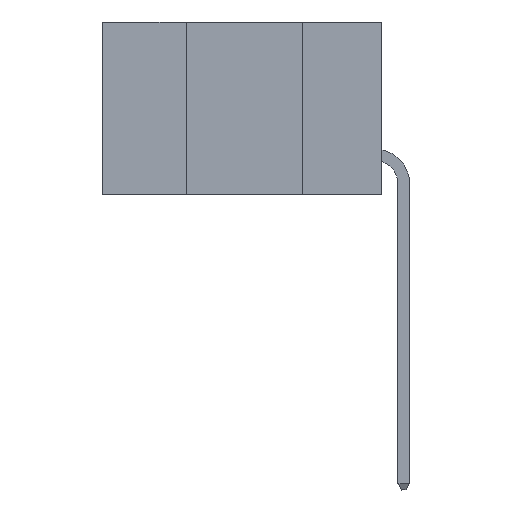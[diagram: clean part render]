
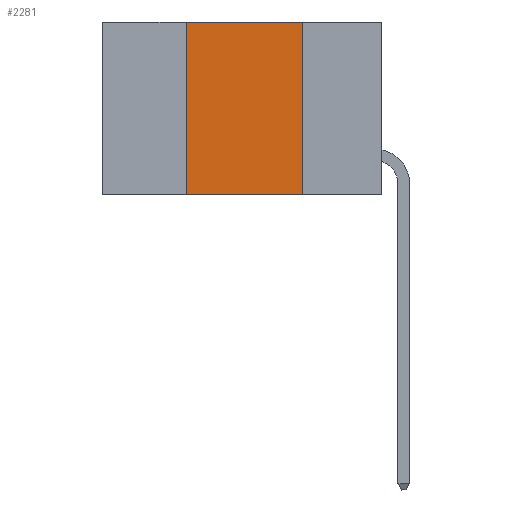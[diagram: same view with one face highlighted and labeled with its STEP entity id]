
A CAD part, left-side view. The second image highlights one B-rep face of the part: STEP entity #2281.
In plain terms, the highlighted planar face has unit normal (-1, 0, 0).
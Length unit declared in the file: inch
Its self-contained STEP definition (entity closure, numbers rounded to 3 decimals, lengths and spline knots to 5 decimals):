
#47 = EDGE_CURVE ( 'NONE', #2455, #6100, #1734, .T. ) ;
#1074 = CARTESIAN_POINT ( 'NONE',  ( 0., 0.6, -0.37 ) ) ;
#1359 = DIRECTION ( 'NONE',  ( 0., 0., 1. ) ) ;
#1734 = LINE ( 'NONE', #14475, #16776 ) ;
#1750 = CARTESIAN_POINT ( 'NONE',  ( 0., 0.17, -0.37 ) ) ;
#1921 = DIRECTION ( 'NONE',  ( 1., 0., 0. ) ) ;
#2025 = VECTOR ( 'NONE', #3415, 39.37008 ) ;
#2040 = DIRECTION ( 'NONE',  ( 0., 0., -1. ) ) ;
#2219 = LINE ( 'NONE', #1074, #16339 ) ;
#2281 = ADVANCED_FACE ( 'NONE', ( #13712 ), #6416, .F. ) ;
#2455 = VERTEX_POINT ( 'NONE', #16823 ) ;
#3310 = VECTOR ( 'NONE', #6194, 39.37008 ) ;
#3415 = DIRECTION ( 'NONE',  ( 0., -1., 0. ) ) ;
#3492 = ORIENTED_EDGE ( 'NONE', *, *, #47, .F. ) ;
#4591 = ORIENTED_EDGE ( 'NONE', *, *, #16192, .T. ) ;
#4711 = ORIENTED_EDGE ( 'NONE', *, *, #14210, .F. ) ;
#5381 = ORIENTED_EDGE ( 'NONE', *, *, #17247, .F. ) ;
#6100 = VERTEX_POINT ( 'NONE', #16876 ) ;
#6194 = DIRECTION ( 'NONE',  ( 0., 0., -1. ) ) ;
#6416 = PLANE ( 'NONE',  #7723 ) ;
#7588 = CARTESIAN_POINT ( 'NONE',  ( 0., 0.17, 0. ) ) ;
#7723 = AXIS2_PLACEMENT_3D ( 'NONE', #16501, #1921, #2040 ) ;
#10730 = CARTESIAN_POINT ( 'NONE',  ( 0., 0.6, 0. ) ) ;
#11298 = DIRECTION ( 'NONE',  ( 0., -1., 0. ) ) ;
#11701 = VERTEX_POINT ( 'NONE', #1750 ) ;
#12304 = LINE ( 'NONE', #10730, #2025 ) ;
#12679 = LINE ( 'NONE', #7588, #3310 ) ;
#13712 = FACE_OUTER_BOUND ( 'NONE', #17482, .T. ) ;
#14210 = EDGE_CURVE ( 'NONE', #6100, #17562, #12304, .T. ) ;
#14475 = CARTESIAN_POINT ( 'NONE',  ( 0., 0.42, 0. ) ) ;
#16192 = EDGE_CURVE ( 'NONE', #2455, #11701, #2219, .T. ) ;
#16339 = VECTOR ( 'NONE', #11298, 39.37008 ) ;
#16501 = CARTESIAN_POINT ( 'NONE',  ( 0., 0.6, 0. ) ) ;
#16776 = VECTOR ( 'NONE', #1359, 39.37008 ) ;
#16823 = CARTESIAN_POINT ( 'NONE',  ( 0., 0.42, -0.37 ) ) ;
#16876 = CARTESIAN_POINT ( 'NONE',  ( 0., 0.42, 0. ) ) ;
#17247 = EDGE_CURVE ( 'NONE', #17562, #11701, #12679, .T. ) ;
#17482 = EDGE_LOOP ( 'NONE', ( #5381, #4711, #3492, #4591 ) ) ;
#17562 = VERTEX_POINT ( 'NONE', #18059 ) ;
#18059 = CARTESIAN_POINT ( 'NONE',  ( 0., 0.17, 0. ) ) ;
